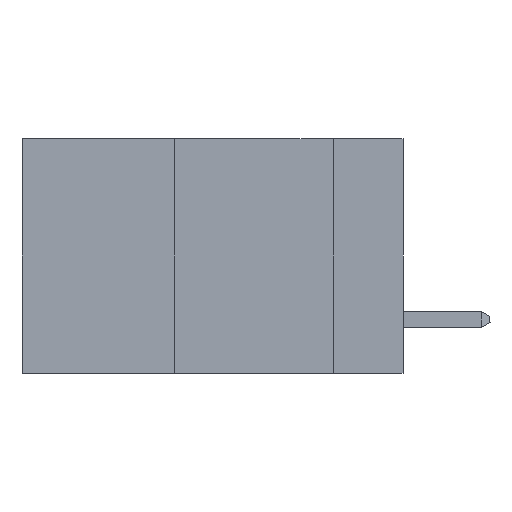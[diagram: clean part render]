
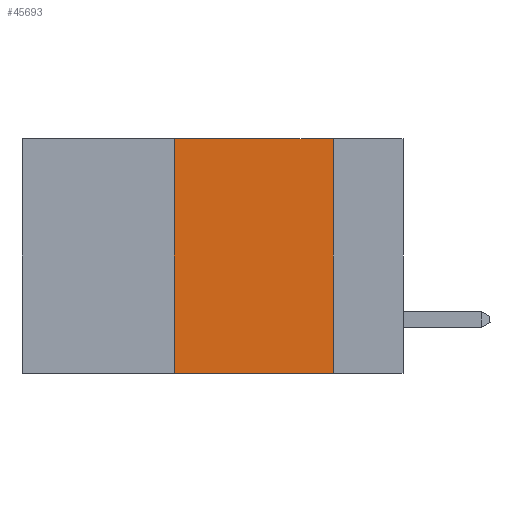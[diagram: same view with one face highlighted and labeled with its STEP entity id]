
A CAD part, left-side view. The second image highlights one B-rep face of the part: STEP entity #45693.
In plain terms, the highlighted planar face has unit normal (-1, 0, 0).
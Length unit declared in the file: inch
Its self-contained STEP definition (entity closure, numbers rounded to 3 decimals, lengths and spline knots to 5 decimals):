
#1307 = VECTOR ( 'NONE', #34945, 39.37008 ) ;
#2013 = DIRECTION ( 'NONE',  ( 0., 0., 1. ) ) ;
#2094 = CARTESIAN_POINT ( 'NONE',  ( 0., 0.36, -0.37 ) ) ;
#3612 = ORIENTED_EDGE ( 'NONE', *, *, #25674, .F. ) ;
#4580 = VECTOR ( 'NONE', #2013, 39.37008 ) ;
#6281 = VECTOR ( 'NONE', #43606, 39.37008 ) ;
#10169 = VECTOR ( 'NONE', #11907, 39.37008 ) ;
#10980 = AXIS2_PLACEMENT_3D ( 'NONE', #31639, #46229, #23528 ) ;
#11553 = VERTEX_POINT ( 'NONE', #16338 ) ;
#11907 = DIRECTION ( 'NONE',  ( 0., -1., 0. ) ) ;
#12379 = EDGE_CURVE ( 'NONE', #28958, #11553, #37300, .T. ) ;
#16283 = ORIENTED_EDGE ( 'NONE', *, *, #26155, .F. ) ;
#16338 = CARTESIAN_POINT ( 'NONE',  ( 0., 0.11, 0. ) ) ;
#20877 = LINE ( 'NONE', #45611, #1307 ) ;
#22087 = FACE_OUTER_BOUND ( 'NONE', #40470, .T. ) ;
#23461 = CARTESIAN_POINT ( 'NONE',  ( 0., 0.6, 0. ) ) ;
#23528 = DIRECTION ( 'NONE',  ( 0., 0., -1. ) ) ;
#24333 = VERTEX_POINT ( 'NONE', #26740 ) ;
#24701 = ORIENTED_EDGE ( 'NONE', *, *, #43854, .T. ) ;
#25674 = EDGE_CURVE ( 'NONE', #38877, #28958, #27681, .T. ) ;
#26155 = EDGE_CURVE ( 'NONE', #11553, #24333, #41525, .T. ) ;
#26740 = CARTESIAN_POINT ( 'NONE',  ( 0., 0.11, -0.37 ) ) ;
#27681 = LINE ( 'NONE', #35575, #4580 ) ;
#28958 = VERTEX_POINT ( 'NONE', #40618 ) ;
#31639 = CARTESIAN_POINT ( 'NONE',  ( 0., 0.6, 0. ) ) ;
#34792 = ORIENTED_EDGE ( 'NONE', *, *, #12379, .F. ) ;
#34945 = DIRECTION ( 'NONE',  ( 0., -1., 0. ) ) ;
#35575 = CARTESIAN_POINT ( 'NONE',  ( 0., 0.36, 0. ) ) ;
#37300 = LINE ( 'NONE', #23461, #10169 ) ;
#38877 = VERTEX_POINT ( 'NONE', #2094 ) ;
#40470 = EDGE_LOOP ( 'NONE', ( #16283, #34792, #3612, #24701 ) ) ;
#40618 = CARTESIAN_POINT ( 'NONE',  ( 0., 0.36, 0. ) ) ;
#41525 = LINE ( 'NONE', #46677, #6281 ) ;
#42515 = PLANE ( 'NONE',  #10980 ) ;
#43606 = DIRECTION ( 'NONE',  ( 0., 0., -1. ) ) ;
#43854 = EDGE_CURVE ( 'NONE', #38877, #24333, #20877, .T. ) ;
#45611 = CARTESIAN_POINT ( 'NONE',  ( 0., 0.6, -0.37 ) ) ;
#45693 = ADVANCED_FACE ( 'NONE', ( #22087 ), #42515, .F. ) ;
#46229 = DIRECTION ( 'NONE',  ( 1., 0., 0. ) ) ;
#46677 = CARTESIAN_POINT ( 'NONE',  ( 0., 0.11, 0. ) ) ;
